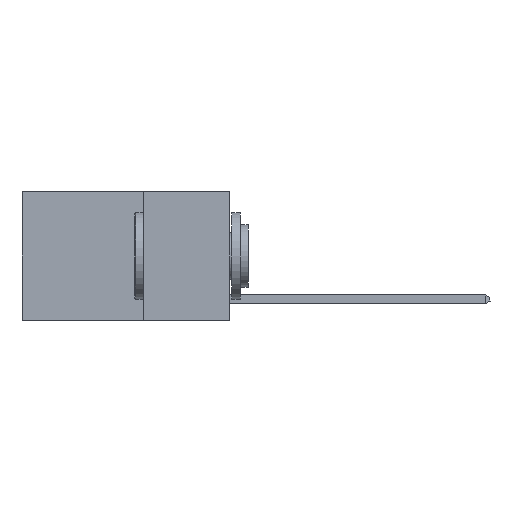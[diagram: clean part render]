
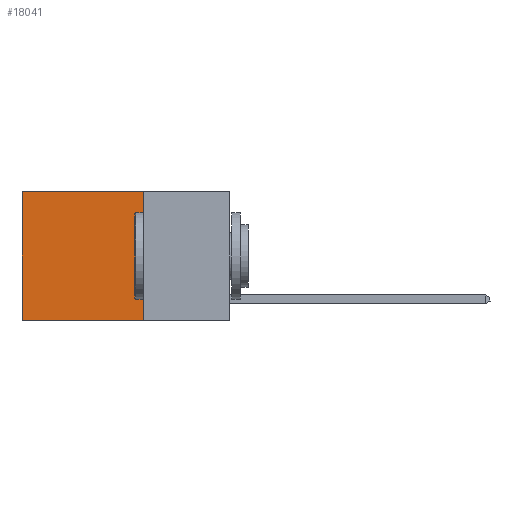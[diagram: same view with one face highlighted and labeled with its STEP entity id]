
A CAD part, left-side view. The second image highlights one B-rep face of the part: STEP entity #18041.
In plain terms, the highlighted planar face has unit normal (-1, 0, 0).
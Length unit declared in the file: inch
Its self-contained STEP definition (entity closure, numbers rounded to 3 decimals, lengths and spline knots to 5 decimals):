
#530 = VERTEX_POINT ( 'NONE', #22286 ) ;
#1408 = EDGE_CURVE ( 'NONE', #21411, #530, #10902, .T. ) ;
#1448 = FACE_OUTER_BOUND ( 'NONE', #26031, .T. ) ;
#1490 = ORIENTED_EDGE ( 'NONE', *, *, #26760, .F. ) ;
#2082 = VECTOR ( 'NONE', #20194, 39.37008 ) ;
#3115 = CARTESIAN_POINT ( 'NONE',  ( 0.2625, 0.25, 0. ) ) ;
#3419 = CARTESIAN_POINT ( 'NONE',  ( 0.2625, 0.6, 0. ) ) ;
#3487 = ORIENTED_EDGE ( 'NONE', *, *, #27208, .T. ) ;
#6357 = AXIS2_PLACEMENT_3D ( 'NONE', #8024, #24669, #14366 ) ;
#7734 = CARTESIAN_POINT ( 'NONE',  ( 0.2625, 0.25, -0.37 ) ) ;
#8024 = CARTESIAN_POINT ( 'NONE',  ( 0.2625, 0.25, 0. ) ) ;
#9620 = VECTOR ( 'NONE', #17123, 39.37008 ) ;
#9717 = LINE ( 'NONE', #3115, #2082 ) ;
#10902 = LINE ( 'NONE', #17181, #16304 ) ;
#11331 = DIRECTION ( 'NONE',  ( 0., 1., 0. ) ) ;
#11342 = DIRECTION ( 'NONE',  ( 0., 0., -1. ) ) ;
#11716 = CARTESIAN_POINT ( 'NONE',  ( 0.2625, 0.25, 0. ) ) ;
#13759 = ORIENTED_EDGE ( 'NONE', *, *, #16465, .T. ) ;
#14366 = DIRECTION ( 'NONE',  ( 0., 0., -1. ) ) ;
#15320 = LINE ( 'NONE', #26569, #9620 ) ;
#15792 = LINE ( 'NONE', #17608, #26167 ) ;
#16304 = VECTOR ( 'NONE', #11331, 39.37008 ) ;
#16465 = EDGE_CURVE ( 'NONE', #20070, #26532, #9717, .T. ) ;
#17123 = DIRECTION ( 'NONE',  ( 0., 0., -1. ) ) ;
#17181 = CARTESIAN_POINT ( 'NONE',  ( 0.2625, 0.25, -0.37 ) ) ;
#17608 = CARTESIAN_POINT ( 'NONE',  ( 0.2625, 0.6, 0. ) ) ;
#18041 = ADVANCED_FACE ( 'NONE', ( #1448 ), #22600, .F. ) ;
#20070 = VERTEX_POINT ( 'NONE', #11716 ) ;
#20194 = DIRECTION ( 'NONE',  ( 0., 1., 0. ) ) ;
#21411 = VERTEX_POINT ( 'NONE', #7734 ) ;
#22286 = CARTESIAN_POINT ( 'NONE',  ( 0.2625, 0.6, -0.37 ) ) ;
#22600 = PLANE ( 'NONE',  #6357 ) ;
#24669 = DIRECTION ( 'NONE',  ( 1., 0., 0. ) ) ;
#26031 = EDGE_LOOP ( 'NONE', ( #3487, #26707, #1490, #13759 ) ) ;
#26167 = VECTOR ( 'NONE', #11342, 39.37008 ) ;
#26532 = VERTEX_POINT ( 'NONE', #3419 ) ;
#26569 = CARTESIAN_POINT ( 'NONE',  ( 0.2625, 0.25, 0. ) ) ;
#26707 = ORIENTED_EDGE ( 'NONE', *, *, #1408, .F. ) ;
#26760 = EDGE_CURVE ( 'NONE', #20070, #21411, #15320, .T. ) ;
#27208 = EDGE_CURVE ( 'NONE', #26532, #530, #15792, .T. ) ;
